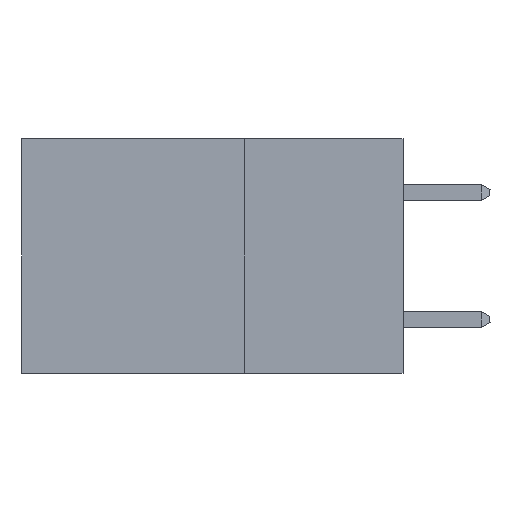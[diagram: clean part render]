
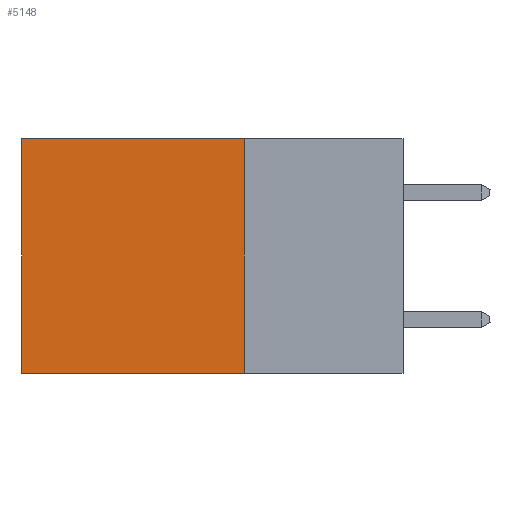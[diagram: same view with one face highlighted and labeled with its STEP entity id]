
A CAD part, left-side view. The second image highlights one B-rep face of the part: STEP entity #5148.
In plain terms, the highlighted planar face has unit normal (-1, 0, 0).
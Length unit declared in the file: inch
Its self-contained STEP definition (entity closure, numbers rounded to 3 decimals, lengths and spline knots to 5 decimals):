
#1627 = DIRECTION ( 'NONE',  ( 1., 0., 0. ) ) ;
#1821 = DIRECTION ( 'NONE',  ( 0., 1., 0. ) ) ;
#2433 = VECTOR ( 'NONE', #15569, 39.37008 ) ;
#3286 = CARTESIAN_POINT ( 'NONE',  ( 0.2875, 0.25, 0. ) ) ;
#4548 = ORIENTED_EDGE ( 'NONE', *, *, #32239, .F. ) ;
#5148 = ADVANCED_FACE ( 'NONE', ( #10372 ), #12500, .F. ) ;
#7288 = LINE ( 'NONE', #31150, #9411 ) ;
#7584 = EDGE_CURVE ( 'NONE', #33388, #21418, #7288, .T. ) ;
#8396 = VECTOR ( 'NONE', #31909, 39.37008 ) ;
#9411 = VECTOR ( 'NONE', #14654, 39.37008 ) ;
#9621 = DIRECTION ( 'NONE',  ( 0., 0., -1. ) ) ;
#9747 = EDGE_CURVE ( 'NONE', #33388, #22542, #10558, .T. ) ;
#10372 = FACE_OUTER_BOUND ( 'NONE', #33664, .T. ) ;
#10558 = LINE ( 'NONE', #32289, #2433 ) ;
#12500 = PLANE ( 'NONE',  #31191 ) ;
#13265 = ORIENTED_EDGE ( 'NONE', *, *, #9747, .F. ) ;
#13709 = ORIENTED_EDGE ( 'NONE', *, *, #18229, .T. ) ;
#13768 = VECTOR ( 'NONE', #1821, 39.37008 ) ;
#14654 = DIRECTION ( 'NONE',  ( 0., 1., 0. ) ) ;
#15569 = DIRECTION ( 'NONE',  ( 0., 0., -1. ) ) ;
#15661 = LINE ( 'NONE', #19667, #8396 ) ;
#18072 = LINE ( 'NONE', #26291, #13768 ) ;
#18229 = EDGE_CURVE ( 'NONE', #21418, #33787, #15661, .T. ) ;
#19667 = CARTESIAN_POINT ( 'NONE',  ( 0.2875, 0.6, 0. ) ) ;
#21418 = VERTEX_POINT ( 'NONE', #29605 ) ;
#22542 = VERTEX_POINT ( 'NONE', #26181 ) ;
#26181 = CARTESIAN_POINT ( 'NONE',  ( 0.2875, 0.25, -0.37 ) ) ;
#26291 = CARTESIAN_POINT ( 'NONE',  ( 0.2875, 0.25, -0.37 ) ) ;
#27399 = CARTESIAN_POINT ( 'NONE',  ( 0.2875, 0.6, -0.37 ) ) ;
#28736 = CARTESIAN_POINT ( 'NONE',  ( 0.2875, 0.25, 0. ) ) ;
#29605 = CARTESIAN_POINT ( 'NONE',  ( 0.2875, 0.6, 0. ) ) ;
#31150 = CARTESIAN_POINT ( 'NONE',  ( 0.2875, 0.25, 0. ) ) ;
#31191 = AXIS2_PLACEMENT_3D ( 'NONE', #28736, #1627, #9621 ) ;
#31909 = DIRECTION ( 'NONE',  ( 0., 0., -1. ) ) ;
#32197 = ORIENTED_EDGE ( 'NONE', *, *, #7584, .T. ) ;
#32239 = EDGE_CURVE ( 'NONE', #22542, #33787, #18072, .T. ) ;
#32289 = CARTESIAN_POINT ( 'NONE',  ( 0.2875, 0.25, 0. ) ) ;
#33388 = VERTEX_POINT ( 'NONE', #3286 ) ;
#33664 = EDGE_LOOP ( 'NONE', ( #13709, #4548, #13265, #32197 ) ) ;
#33787 = VERTEX_POINT ( 'NONE', #27399 ) ;
